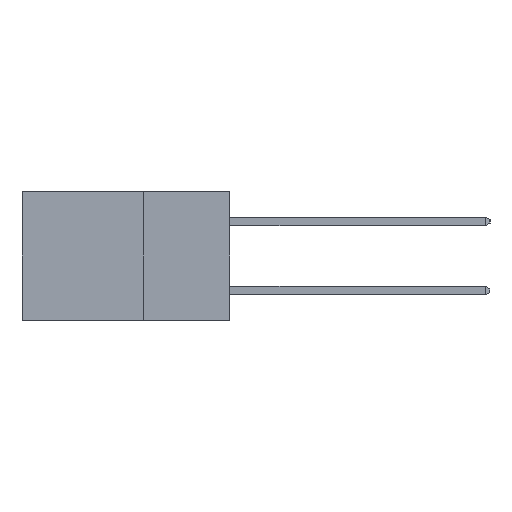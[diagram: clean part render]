
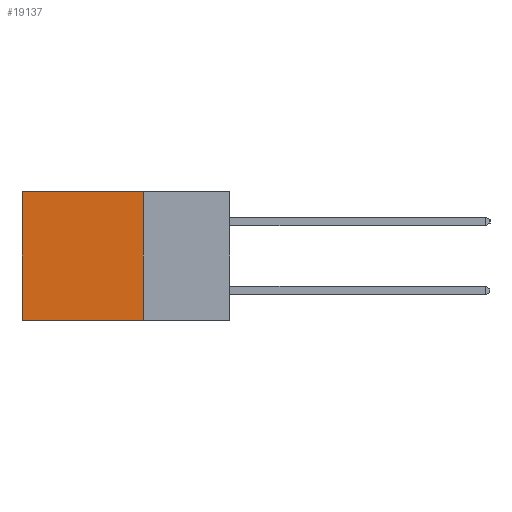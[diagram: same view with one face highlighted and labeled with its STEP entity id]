
A CAD part, left-side view. The second image highlights one B-rep face of the part: STEP entity #19137.
In plain terms, the highlighted planar face has unit normal (-1, 0, 0).
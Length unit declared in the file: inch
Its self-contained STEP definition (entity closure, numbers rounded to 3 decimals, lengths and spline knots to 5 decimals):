
#389 = VERTEX_POINT ( 'NONE', #29381 ) ;
#986 = VERTEX_POINT ( 'NONE', #28234 ) ;
#3146 = EDGE_CURVE ( 'NONE', #18741, #986, #14413, .T. ) ;
#4203 = CARTESIAN_POINT ( 'NONE',  ( 0.298, 0.25, 0. ) ) ;
#4213 = AXIS2_PLACEMENT_3D ( 'NONE', #4203, #6589, #22969 ) ;
#4343 = ORIENTED_EDGE ( 'NONE', *, *, #3146, .T. ) ;
#4379 = EDGE_LOOP ( 'NONE', ( #7866, #13586, #5098, #4343 ) ) ;
#4663 = CARTESIAN_POINT ( 'NONE',  ( 0.298, 0.25, -0.37 ) ) ;
#4836 = LINE ( 'NONE', #4663, #11119 ) ;
#5098 = ORIENTED_EDGE ( 'NONE', *, *, #13385, .F. ) ;
#5158 = CARTESIAN_POINT ( 'NONE',  ( 0.298, 0.25, 0. ) ) ;
#6589 = DIRECTION ( 'NONE',  ( 1., 0., 0. ) ) ;
#6737 = VERTEX_POINT ( 'NONE', #29284 ) ;
#7866 = ORIENTED_EDGE ( 'NONE', *, *, #13272, .T. ) ;
#9464 = LINE ( 'NONE', #15271, #27327 ) ;
#11119 = VECTOR ( 'NONE', #21054, 39.37008 ) ;
#12737 = LINE ( 'NONE', #29551, #29836 ) ;
#13272 = EDGE_CURVE ( 'NONE', #986, #389, #9464, .T. ) ;
#13385 = EDGE_CURVE ( 'NONE', #18741, #6737, #12737, .T. ) ;
#13586 = ORIENTED_EDGE ( 'NONE', *, *, #30228, .F. ) ;
#14413 = LINE ( 'NONE', #15729, #19858 ) ;
#14714 = DIRECTION ( 'NONE',  ( 0., 1., 0. ) ) ;
#15271 = CARTESIAN_POINT ( 'NONE',  ( 0.298, 0.6, 0. ) ) ;
#15729 = CARTESIAN_POINT ( 'NONE',  ( 0.298, 0.25, 0. ) ) ;
#17583 = DIRECTION ( 'NONE',  ( 0., 0., -1. ) ) ;
#17982 = DIRECTION ( 'NONE',  ( 0., 0., -1. ) ) ;
#18278 = PLANE ( 'NONE',  #4213 ) ;
#18741 = VERTEX_POINT ( 'NONE', #5158 ) ;
#19137 = ADVANCED_FACE ( 'NONE', ( #24434 ), #18278, .F. ) ;
#19858 = VECTOR ( 'NONE', #14714, 39.37008 ) ;
#21054 = DIRECTION ( 'NONE',  ( 0., 1., 0. ) ) ;
#22969 = DIRECTION ( 'NONE',  ( 0., 0., -1. ) ) ;
#24434 = FACE_OUTER_BOUND ( 'NONE', #4379, .T. ) ;
#27327 = VECTOR ( 'NONE', #17583, 39.37008 ) ;
#28234 = CARTESIAN_POINT ( 'NONE',  ( 0.298, 0.6, 0. ) ) ;
#29284 = CARTESIAN_POINT ( 'NONE',  ( 0.298, 0.25, -0.37 ) ) ;
#29381 = CARTESIAN_POINT ( 'NONE',  ( 0.298, 0.6, -0.37 ) ) ;
#29551 = CARTESIAN_POINT ( 'NONE',  ( 0.298, 0.25, 0. ) ) ;
#29836 = VECTOR ( 'NONE', #17982, 39.37008 ) ;
#30228 = EDGE_CURVE ( 'NONE', #6737, #389, #4836, .T. ) ;
